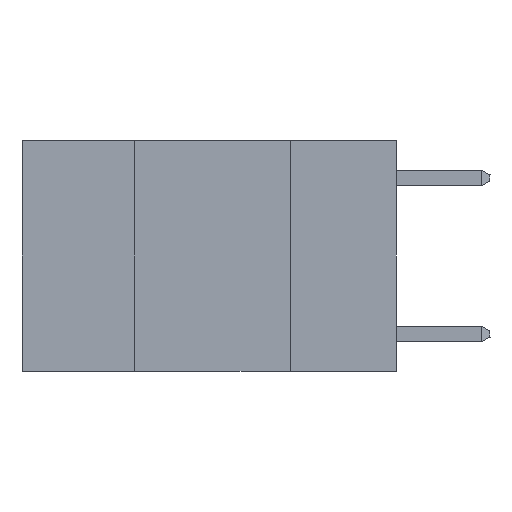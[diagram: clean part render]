
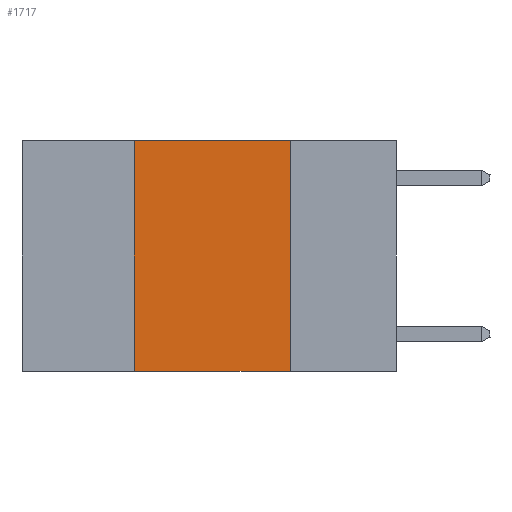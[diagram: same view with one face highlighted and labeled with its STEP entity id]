
A CAD part, left-side view. The second image highlights one B-rep face of the part: STEP entity #1717.
In plain terms, the highlighted planar face has unit normal (-1, 0, 0).
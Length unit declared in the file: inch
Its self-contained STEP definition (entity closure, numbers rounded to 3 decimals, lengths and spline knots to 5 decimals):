
#317 = VECTOR ( 'NONE', #1142, 39.37008 ) ;
#1142 = DIRECTION ( 'NONE',  ( 0., -1., 0. ) ) ;
#1616 = VERTEX_POINT ( 'NONE', #20677 ) ;
#1717 = ADVANCED_FACE ( 'NONE', ( #18073 ), #10320, .F. ) ;
#1767 = DIRECTION ( 'NONE',  ( 0., -1., 0. ) ) ;
#1837 = VERTEX_POINT ( 'NONE', #2986 ) ;
#2986 = CARTESIAN_POINT ( 'NONE',  ( 0., 0.42, 0. ) ) ;
#3266 = EDGE_CURVE ( 'NONE', #1837, #9874, #15227, .T. ) ;
#3313 = CARTESIAN_POINT ( 'NONE',  ( 0., 0.6, 0. ) ) ;
#4569 = EDGE_CURVE ( 'NONE', #9874, #20019, #16480, .T. ) ;
#4707 = LINE ( 'NONE', #12729, #317 ) ;
#4729 = ORIENTED_EDGE ( 'NONE', *, *, #4569, .F. ) ;
#5241 = CARTESIAN_POINT ( 'NONE',  ( 0., 0.6, 0. ) ) ;
#6363 = CARTESIAN_POINT ( 'NONE',  ( 0., 0.17, 0. ) ) ;
#6525 = DIRECTION ( 'NONE',  ( 1., 0., 0. ) ) ;
#8989 = DIRECTION ( 'NONE',  ( 0., 0., 1. ) ) ;
#9869 = CARTESIAN_POINT ( 'NONE',  ( 0., 0.17, -0.37 ) ) ;
#9874 = VERTEX_POINT ( 'NONE', #20376 ) ;
#10320 = PLANE ( 'NONE',  #11964 ) ;
#11587 = ORIENTED_EDGE ( 'NONE', *, *, #14763, .F. ) ;
#11964 = AXIS2_PLACEMENT_3D ( 'NONE', #3313, #6525, #19678 ) ;
#12466 = ORIENTED_EDGE ( 'NONE', *, *, #16675, .T. ) ;
#12729 = CARTESIAN_POINT ( 'NONE',  ( 0., 0.6, -0.37 ) ) ;
#13848 = CARTESIAN_POINT ( 'NONE',  ( 0., 0.42, 0. ) ) ;
#13920 = VECTOR ( 'NONE', #1767, 39.37008 ) ;
#14740 = DIRECTION ( 'NONE',  ( 0., 0., -1. ) ) ;
#14763 = EDGE_CURVE ( 'NONE', #1616, #1837, #18709, .T. ) ;
#15227 = LINE ( 'NONE', #5241, #13920 ) ;
#15907 = ORIENTED_EDGE ( 'NONE', *, *, #3266, .F. ) ;
#16480 = LINE ( 'NONE', #6363, #18797 ) ;
#16675 = EDGE_CURVE ( 'NONE', #1616, #20019, #4707, .T. ) ;
#17307 = EDGE_LOOP ( 'NONE', ( #4729, #15907, #11587, #12466 ) ) ;
#18073 = FACE_OUTER_BOUND ( 'NONE', #17307, .T. ) ;
#18709 = LINE ( 'NONE', #13848, #20526 ) ;
#18797 = VECTOR ( 'NONE', #14740, 39.37008 ) ;
#19678 = DIRECTION ( 'NONE',  ( 0., 0., -1. ) ) ;
#20019 = VERTEX_POINT ( 'NONE', #9869 ) ;
#20376 = CARTESIAN_POINT ( 'NONE',  ( 0., 0.17, 0. ) ) ;
#20526 = VECTOR ( 'NONE', #8989, 39.37008 ) ;
#20677 = CARTESIAN_POINT ( 'NONE',  ( 0., 0.42, -0.37 ) ) ;
